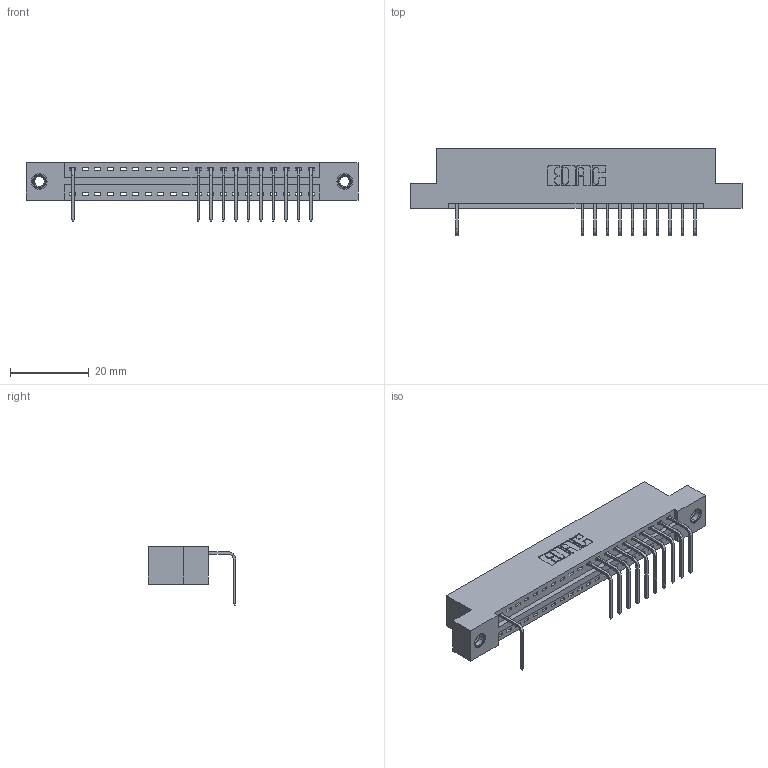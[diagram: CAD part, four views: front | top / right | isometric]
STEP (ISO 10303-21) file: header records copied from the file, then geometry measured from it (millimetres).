
FILE_DESCRIPTION (( 'STEP AP203' ), '1' );
FILE_NAME ('346-020-558-107.STEP', '2018-08-20T22:07:37', ( '' ), ( '' ), 'SwSTEP 2.0', 'SolidWorks 2016', '' );
FILE_SCHEMA (( 'CONFIG_CONTROL_DESIGN' ));
Length unit declared in the file: inch
Products named in the file (4): 346 Part_Flush Mounting Lugs - 0.156 Dia-TI; 345-292-001_558 Tail - 2; 345-250-001_345-250-005-103; 346-020-558-107
Assembly tree (14 placements, depth 2):
  346-020-558-107
    346 Part_Flush Mounting Lugs - 0.156 Dia-TI
    345-292-001_558 Tail - 2  x11
    345-250-001_345-250-005-103  x2
Bounding box: 84.07 x 22.16 x 14.73 mm (x, y, z)
Volume: 7816.4 mm3; surface area: 9231.5 mm2
Topology: 14 solids, 14 shells, 950 faces, 2845 edges, 1874 vertices
Faces by surface type: plane 660, cylinder 274, cone 12, torus 4
Entity records: 16356 total; most frequent: CARTESIAN_POINT 2834, ORIENTED_EDGE 2790, DIRECTION 2543, EDGE_CURVE 1395, VECTOR 1163, LINE 1163, VERTEX_POINT 924, AXIS2_PLACEMENT_3D 690
